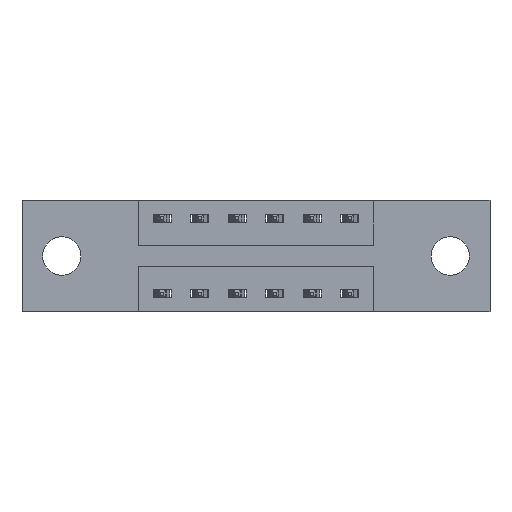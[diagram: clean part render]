
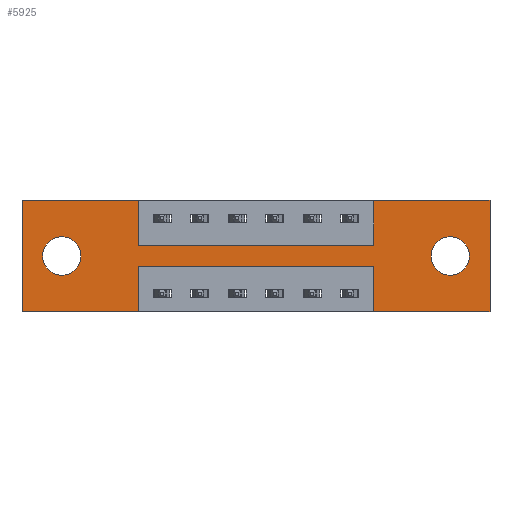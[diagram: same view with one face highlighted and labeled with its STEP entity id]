
A CAD part, front view. The second image highlights one B-rep face of the part: STEP entity #5925.
In plain terms, the highlighted planar face has unit normal (0, -1, 0).
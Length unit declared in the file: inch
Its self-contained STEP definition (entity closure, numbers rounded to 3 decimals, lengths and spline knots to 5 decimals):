
#29 = CARTESIAN_POINT ( 'NONE',  ( 1.4275, 0., -0.249 ) ) ;
#67 = DIRECTION ( 'NONE',  ( 0., 1., 0. ) ) ;
#83 = CARTESIAN_POINT ( 'NONE',  ( 0.1325, 0., -0.249 ) ) ;
#119 = ORIENTED_EDGE ( 'NONE', *, *, #3683, .F. ) ;
#243 = VERTEX_POINT ( 'NONE', #6820 ) ;
#253 = VERTEX_POINT ( 'NONE', #1324 ) ;
#339 = CARTESIAN_POINT ( 'NONE',  ( 0., 0., -0.37 ) ) ;
#366 = CARTESIAN_POINT ( 'NONE',  ( 1.56, 0., 0. ) ) ;
#384 = CIRCLE ( 'NONE', #3239, 0.064 ) ;
#403 = AXIS2_PLACEMENT_3D ( 'NONE', #6743, #2695, #685 ) ;
#478 = CARTESIAN_POINT ( 'NONE',  ( 0., 0., -0.37 ) ) ;
#527 = VECTOR ( 'NONE', #6689, 39.37008 ) ;
#550 = VERTEX_POINT ( 'NONE', #5120 ) ;
#553 = ORIENTED_EDGE ( 'NONE', *, *, #1184, .F. ) ;
#627 = LINE ( 'NONE', #4832, #7657 ) ;
#685 = DIRECTION ( 'NONE',  ( 0., 0., 1. ) ) ;
#701 = EDGE_CURVE ( 'NONE', #6766, #4406, #4403, .T. ) ;
#761 = ORIENTED_EDGE ( 'NONE', *, *, #701, .F. ) ;
#855 = ORIENTED_EDGE ( 'NONE', *, *, #2360, .F. ) ;
#889 = LINE ( 'NONE', #1337, #8108 ) ;
#958 = EDGE_CURVE ( 'NONE', #4829, #253, #3854, .T. ) ;
#1184 = EDGE_CURVE ( 'NONE', #4863, #243, #627, .T. ) ;
#1190 = CARTESIAN_POINT ( 'NONE',  ( 0.3875, 0., 0. ) ) ;
#1230 = EDGE_CURVE ( 'NONE', #5130, #6331, #6069, .T. ) ;
#1324 = CARTESIAN_POINT ( 'NONE',  ( 0.3875, 0., -0.15 ) ) ;
#1337 = CARTESIAN_POINT ( 'NONE',  ( 1.1725, 0., 0. ) ) ;
#1460 = FACE_BOUND ( 'NONE', #5895, .T. ) ;
#1530 = DIRECTION ( 'NONE',  ( 0., 0., -1. ) ) ;
#1615 = VECTOR ( 'NONE', #1530, 39.37008 ) ;
#1789 = VECTOR ( 'NONE', #4177, 39.37008 ) ;
#1955 = CARTESIAN_POINT ( 'NONE',  ( 0., 0., -0.37 ) ) ;
#2011 = DIRECTION ( 'NONE',  ( 0., 1., 0. ) ) ;
#2032 = CARTESIAN_POINT ( 'NONE',  ( 1.4275, 0., -0.185 ) ) ;
#2066 = EDGE_CURVE ( 'NONE', #4764, #2420, #7217, .T. ) ;
#2105 = CARTESIAN_POINT ( 'NONE',  ( 0.3875, 0., -0.22 ) ) ;
#2164 = VERTEX_POINT ( 'NONE', #2958 ) ;
#2203 = ORIENTED_EDGE ( 'NONE', *, *, #3789, .F. ) ;
#2325 = FACE_OUTER_BOUND ( 'NONE', #3904, .T. ) ;
#2360 = EDGE_CURVE ( 'NONE', #550, #7562, #3618, .T. ) ;
#2409 = ORIENTED_EDGE ( 'NONE', *, *, #958, .F. ) ;
#2420 = VERTEX_POINT ( 'NONE', #83 ) ;
#2438 = LINE ( 'NONE', #1955, #6788 ) ;
#2498 = LINE ( 'NONE', #7768, #8080 ) ;
#2534 = EDGE_CURVE ( 'NONE', #243, #5130, #2438, .T. ) ;
#2592 = DIRECTION ( 'NONE',  ( 0., 0., -1. ) ) ;
#2695 = DIRECTION ( 'NONE',  ( 0., 1., 0. ) ) ;
#2754 = CARTESIAN_POINT ( 'NONE',  ( 1.56, 0., -0.37 ) ) ;
#2794 = CARTESIAN_POINT ( 'NONE',  ( 1.4275, 0., -0.185 ) ) ;
#2795 = CARTESIAN_POINT ( 'NONE',  ( 0.3875, 0., 0. ) ) ;
#2887 = DIRECTION ( 'NONE',  ( 0., 0., 1. ) ) ;
#2950 = EDGE_CURVE ( 'NONE', #3070, #3236, #7820, .T. ) ;
#2954 = VECTOR ( 'NONE', #6629, 39.37008 ) ;
#2958 = CARTESIAN_POINT ( 'NONE',  ( 1.1725, 0., -0.15 ) ) ;
#3020 = VERTEX_POINT ( 'NONE', #7428 ) ;
#3070 = VERTEX_POINT ( 'NONE', #29 ) ;
#3202 = EDGE_CURVE ( 'NONE', #6331, #4829, #5827, .T. ) ;
#3236 = VERTEX_POINT ( 'NONE', #4756 ) ;
#3239 = AXIS2_PLACEMENT_3D ( 'NONE', #2032, #6787, #8115 ) ;
#3304 = ORIENTED_EDGE ( 'NONE', *, *, #1230, .F. ) ;
#3353 = DIRECTION ( 'NONE',  ( 0., 0., 1. ) ) ;
#3382 = CARTESIAN_POINT ( 'NONE',  ( 0.1325, 0., -0.121 ) ) ;
#3445 = CARTESIAN_POINT ( 'NONE',  ( 0., 0., -0.37 ) ) ;
#3484 = AXIS2_PLACEMENT_3D ( 'NONE', #2794, #67, #6929 ) ;
#3618 = LINE ( 'NONE', #6159, #1789 ) ;
#3683 = EDGE_CURVE ( 'NONE', #253, #2164, #6714, .T. ) ;
#3769 = DIRECTION ( 'NONE',  ( 1., 0., 0. ) ) ;
#3782 = AXIS2_PLACEMENT_3D ( 'NONE', #3445, #4145, #7733 ) ;
#3789 = EDGE_CURVE ( 'NONE', #7562, #6766, #8785, .T. ) ;
#3854 = LINE ( 'NONE', #1190, #527 ) ;
#3904 = EDGE_LOOP ( 'NONE', ( #553, #3983, #8457, #761, #2203, #855, #7177, #119, #2409, #8431, #3304, #4281 ) ) ;
#3914 = ORIENTED_EDGE ( 'NONE', *, *, #5394, .T. ) ;
#3983 = ORIENTED_EDGE ( 'NONE', *, *, #6430, .F. ) ;
#4087 = CARTESIAN_POINT ( 'NONE',  ( 0.3875, 0., -0.15 ) ) ;
#4093 = DIRECTION ( 'NONE',  ( 0., 0., 1. ) ) ;
#4145 = DIRECTION ( 'NONE',  ( 0., -1., 0. ) ) ;
#4177 = DIRECTION ( 'NONE',  ( 1., 0., 0. ) ) ;
#4252 = CARTESIAN_POINT ( 'NONE',  ( 1.1725, 0., -0.37 ) ) ;
#4281 = ORIENTED_EDGE ( 'NONE', *, *, #2534, .F. ) ;
#4403 = LINE ( 'NONE', #478, #8471 ) ;
#4406 = VERTEX_POINT ( 'NONE', #4252 ) ;
#4685 = EDGE_CURVE ( 'NONE', #2420, #4764, #8259, .T. ) ;
#4755 = LINE ( 'NONE', #5286, #2954 ) ;
#4756 = CARTESIAN_POINT ( 'NONE',  ( 1.4275, 0., -0.121 ) ) ;
#4764 = VERTEX_POINT ( 'NONE', #3382 ) ;
#4829 = VERTEX_POINT ( 'NONE', #2795 ) ;
#4832 = CARTESIAN_POINT ( 'NONE',  ( 0.3875, 0., -0.37 ) ) ;
#4863 = VERTEX_POINT ( 'NONE', #2105 ) ;
#5120 = CARTESIAN_POINT ( 'NONE',  ( 1.1725, 0., 0. ) ) ;
#5130 = VERTEX_POINT ( 'NONE', #339 ) ;
#5190 = DIRECTION ( 'NONE',  ( 0., 0., 1. ) ) ;
#5286 = CARTESIAN_POINT ( 'NONE',  ( 0.3875, 0., -0.22 ) ) ;
#5326 = DIRECTION ( 'NONE',  ( 1., 0., 0. ) ) ;
#5386 = DIRECTION ( 'NONE',  ( -1., 0., 0. ) ) ;
#5394 = EDGE_CURVE ( 'NONE', #3236, #3070, #384, .T. ) ;
#5490 = ORIENTED_EDGE ( 'NONE', *, *, #2066, .T. ) ;
#5827 = LINE ( 'NONE', #7798, #6474 ) ;
#5895 = EDGE_LOOP ( 'NONE', ( #5490, #7564 ) ) ;
#5925 = ADVANCED_FACE ( 'NONE', ( #6997, #1460, #2325 ), #8136, .T. ) ;
#6069 = LINE ( 'NONE', #8279, #8674 ) ;
#6159 = CARTESIAN_POINT ( 'NONE',  ( 0., 0., 0. ) ) ;
#6331 = VERTEX_POINT ( 'NONE', #7058 ) ;
#6386 = CARTESIAN_POINT ( 'NONE',  ( 1.56, 0., 0. ) ) ;
#6430 = EDGE_CURVE ( 'NONE', #3020, #4863, #4755, .T. ) ;
#6474 = VECTOR ( 'NONE', #3769, 39.37008 ) ;
#6629 = DIRECTION ( 'NONE',  ( -1., 0., 0. ) ) ;
#6689 = DIRECTION ( 'NONE',  ( 0., 0., -1. ) ) ;
#6714 = LINE ( 'NONE', #4087, #8676 ) ;
#6743 = CARTESIAN_POINT ( 'NONE',  ( 0.1325, 0., -0.185 ) ) ;
#6747 = ORIENTED_EDGE ( 'NONE', *, *, #2950, .T. ) ;
#6766 = VERTEX_POINT ( 'NONE', #2754 ) ;
#6787 = DIRECTION ( 'NONE',  ( 0., 1., 0. ) ) ;
#6788 = VECTOR ( 'NONE', #5386, 39.37008 ) ;
#6820 = CARTESIAN_POINT ( 'NONE',  ( 0.3875, 0., -0.37 ) ) ;
#6929 = DIRECTION ( 'NONE',  ( 0., 0., -1. ) ) ;
#6997 = FACE_BOUND ( 'NONE', #7770, .T. ) ;
#7058 = CARTESIAN_POINT ( 'NONE',  ( 0., 0., 0. ) ) ;
#7177 = ORIENTED_EDGE ( 'NONE', *, *, #7320, .F. ) ;
#7217 = CIRCLE ( 'NONE', #403, 0.064 ) ;
#7320 = EDGE_CURVE ( 'NONE', #2164, #550, #889, .T. ) ;
#7352 = CARTESIAN_POINT ( 'NONE',  ( 0.1325, 0., -0.185 ) ) ;
#7428 = CARTESIAN_POINT ( 'NONE',  ( 1.1725, 0., -0.22 ) ) ;
#7562 = VERTEX_POINT ( 'NONE', #366 ) ;
#7564 = ORIENTED_EDGE ( 'NONE', *, *, #4685, .T. ) ;
#7657 = VECTOR ( 'NONE', #2592, 39.37008 ) ;
#7733 = DIRECTION ( 'NONE',  ( 0., 0., -1. ) ) ;
#7768 = CARTESIAN_POINT ( 'NONE',  ( 1.1725, 0., -0.37 ) ) ;
#7770 = EDGE_LOOP ( 'NONE', ( #3914, #6747 ) ) ;
#7798 = CARTESIAN_POINT ( 'NONE',  ( 0., 0., 0. ) ) ;
#7820 = CIRCLE ( 'NONE', #3484, 0.064 ) ;
#8080 = VECTOR ( 'NONE', #2887, 39.37008 ) ;
#8108 = VECTOR ( 'NONE', #4093, 39.37008 ) ;
#8115 = DIRECTION ( 'NONE',  ( 0., 0., -1. ) ) ;
#8136 = PLANE ( 'NONE',  #3782 ) ;
#8259 = CIRCLE ( 'NONE', #8566, 0.064 ) ;
#8279 = CARTESIAN_POINT ( 'NONE',  ( 0., 0., 0. ) ) ;
#8431 = ORIENTED_EDGE ( 'NONE', *, *, #3202, .F. ) ;
#8457 = ORIENTED_EDGE ( 'NONE', *, *, #8575, .F. ) ;
#8471 = VECTOR ( 'NONE', #8523, 39.37008 ) ;
#8523 = DIRECTION ( 'NONE',  ( -1., 0., 0. ) ) ;
#8566 = AXIS2_PLACEMENT_3D ( 'NONE', #7352, #2011, #3353 ) ;
#8575 = EDGE_CURVE ( 'NONE', #4406, #3020, #2498, .T. ) ;
#8674 = VECTOR ( 'NONE', #5190, 39.37008 ) ;
#8676 = VECTOR ( 'NONE', #5326, 39.37008 ) ;
#8785 = LINE ( 'NONE', #6386, #1615 ) ;
